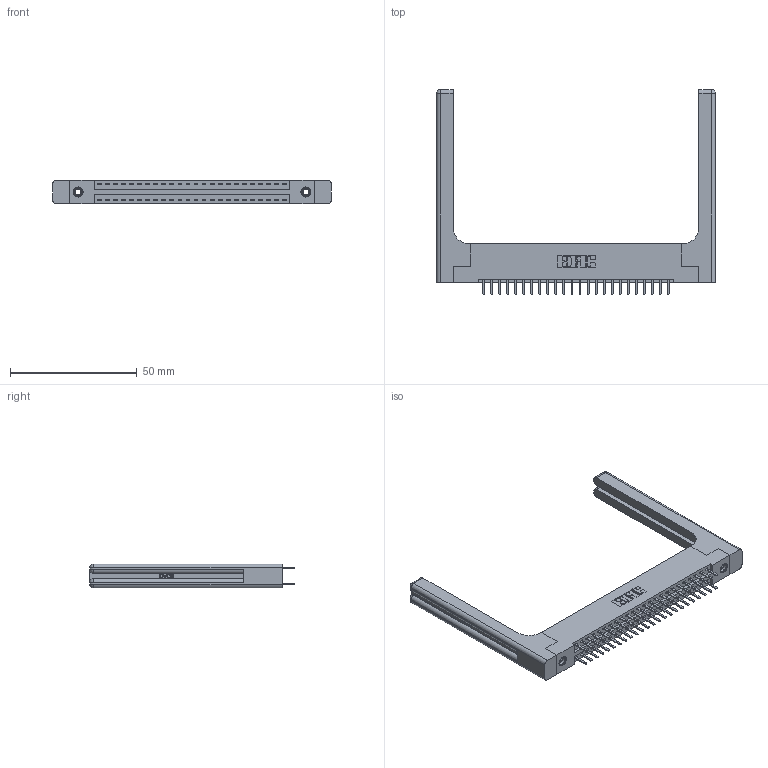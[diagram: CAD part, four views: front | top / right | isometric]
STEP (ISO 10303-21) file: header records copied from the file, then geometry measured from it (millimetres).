
FILE_DESCRIPTION (( 'STEP AP203' ), '1' );
FILE_NAME ('346-048-520-258.STEP', '2022-05-20T21:01:12', ( '' ), ( '' ), 'SwSTEP 2.0', 'SolidWorks 2020', '' );
FILE_SCHEMA (( 'CONFIG_CONTROL_DESIGN' ));
Length unit declared in the file: inch
Products named in the file (5): 345-250-001_345-250-001-102; 346-220-058_345-220-058; 346-048-520-258; 346 Part_Flush Mounting Lugs - 0.156 Dia-TH; 345-292-001_345-293-120
Assembly tree (53 placements, depth 2):
  346-048-520-258
    346 Part_Flush Mounting Lugs - 0.156 Dia-TH
    345-292-001_345-293-120  x48
    345-250-001_345-250-001-102  x2
    346-220-058_345-220-058  x2
Bounding box: 110.26 x 80.98 x 9.4 mm (x, y, z)
Volume: 18067.1 mm3; surface area: 19208.1 mm2
Topology: 53 solids, 53 shells, 3080 faces, 8855 edges, 5754 vertices
Faces by surface type: plane 2014, cylinder 1006, bspline 36, cone 12, sphere 8, torus 4
Entity records: 23798 total; most frequent: CARTESIAN_POINT 4971, ORIENTED_EDGE 3688, DIRECTION 3352, EDGE_CURVE 1844, LINE 1520, VECTOR 1520, VERTEX_POINT 1218, AXIS2_PLACEMENT_3D 916
